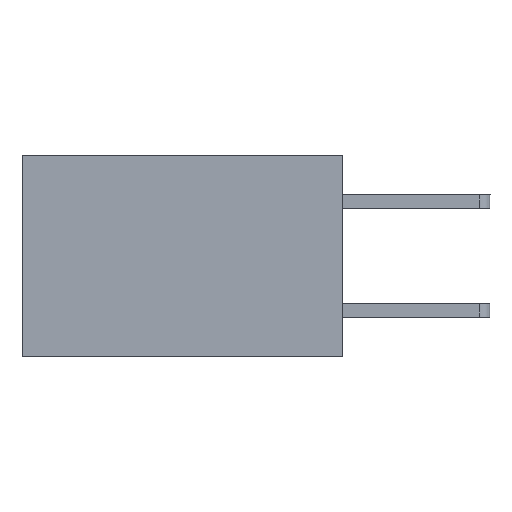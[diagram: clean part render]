
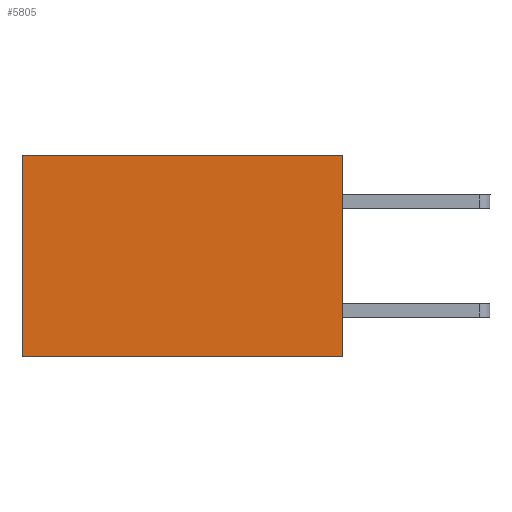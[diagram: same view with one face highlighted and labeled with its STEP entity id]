
A CAD part, left-side view. The second image highlights one B-rep face of the part: STEP entity #5805.
In plain terms, the highlighted planar face has unit normal (-1, 0, 0).
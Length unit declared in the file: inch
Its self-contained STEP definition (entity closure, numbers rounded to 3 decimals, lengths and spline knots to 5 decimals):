
#429 = CARTESIAN_POINT ( 'NONE',  ( 0.277, 0., -0.37 ) ) ;
#492 = ORIENTED_EDGE ( 'NONE', *, *, #6072, .F. ) ;
#549 = VECTOR ( 'NONE', #8525, 39.37008 ) ;
#1280 = CARTESIAN_POINT ( 'NONE',  ( 0.277, 0.59, -0.37 ) ) ;
#1500 = EDGE_CURVE ( 'NONE', #8475, #5527, #6149, .T. ) ;
#2199 = CARTESIAN_POINT ( 'NONE',  ( 0.277, 0.59, 0. ) ) ;
#2202 = CARTESIAN_POINT ( 'NONE',  ( 0.277, 0., -0.37 ) ) ;
#2227 = CARTESIAN_POINT ( 'NONE',  ( 0.277, 0.59, -0.37 ) ) ;
#2379 = VECTOR ( 'NONE', #8906, 39.37008 ) ;
#2892 = FACE_OUTER_BOUND ( 'NONE', #7564, .T. ) ;
#2919 = ORIENTED_EDGE ( 'NONE', *, *, #1500, .T. ) ;
#3346 = CARTESIAN_POINT ( 'NONE',  ( 0.277, 0., -0.37 ) ) ;
#3410 = ORIENTED_EDGE ( 'NONE', *, *, #7672, .T. ) ;
#3506 = AXIS2_PLACEMENT_3D ( 'NONE', #8437, #9966, #10067 ) ;
#3639 = LINE ( 'NONE', #2202, #8756 ) ;
#3850 = VECTOR ( 'NONE', #9647, 39.37008 ) ;
#4340 = LINE ( 'NONE', #1280, #2379 ) ;
#5282 = PLANE ( 'NONE',  #3506 ) ;
#5527 = VERTEX_POINT ( 'NONE', #2199 ) ;
#5805 = ADVANCED_FACE ( 'NONE', ( #2892 ), #5282, .F. ) ;
#5857 = VERTEX_POINT ( 'NONE', #2227 ) ;
#5934 = DIRECTION ( 'NONE',  ( 0., 0., -1. ) ) ;
#6072 = EDGE_CURVE ( 'NONE', #6100, #5857, #6661, .T. ) ;
#6100 = VERTEX_POINT ( 'NONE', #429 ) ;
#6149 = LINE ( 'NONE', #8667, #549 ) ;
#6661 = LINE ( 'NONE', #3346, #3850 ) ;
#6720 = EDGE_CURVE ( 'NONE', #8475, #6100, #3639, .T. ) ;
#7408 = ORIENTED_EDGE ( 'NONE', *, *, #6720, .F. ) ;
#7564 = EDGE_LOOP ( 'NONE', ( #3410, #492, #7408, #2919 ) ) ;
#7672 = EDGE_CURVE ( 'NONE', #5527, #5857, #4340, .T. ) ;
#8437 = CARTESIAN_POINT ( 'NONE',  ( 0.277, 0., -0.37 ) ) ;
#8475 = VERTEX_POINT ( 'NONE', #8772 ) ;
#8525 = DIRECTION ( 'NONE',  ( 0., 1., 0. ) ) ;
#8667 = CARTESIAN_POINT ( 'NONE',  ( 0.277, 0., 0. ) ) ;
#8756 = VECTOR ( 'NONE', #5934, 39.37008 ) ;
#8772 = CARTESIAN_POINT ( 'NONE',  ( 0.277, 0., 0. ) ) ;
#8906 = DIRECTION ( 'NONE',  ( 0., 0., -1. ) ) ;
#9647 = DIRECTION ( 'NONE',  ( 0., 1., 0. ) ) ;
#9966 = DIRECTION ( 'NONE',  ( 1., 0., 0. ) ) ;
#10067 = DIRECTION ( 'NONE',  ( 0., 0., -1. ) ) ;
